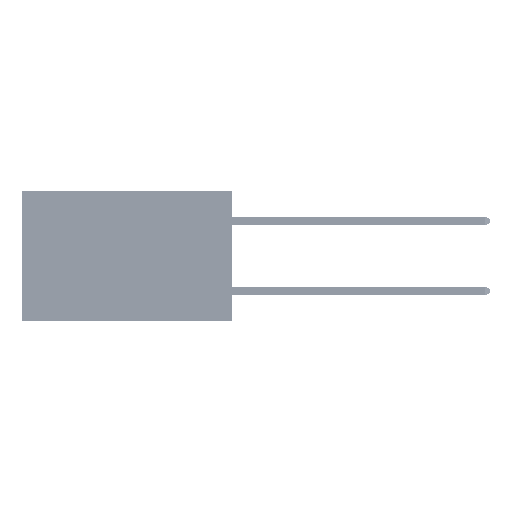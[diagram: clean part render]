
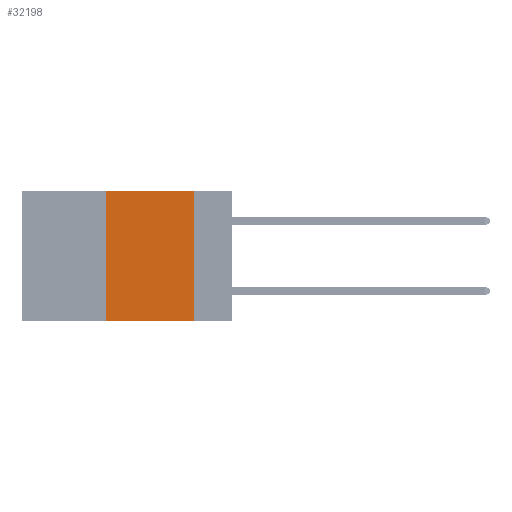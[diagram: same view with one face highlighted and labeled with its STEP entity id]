
A CAD part, left-side view. The second image highlights one B-rep face of the part: STEP entity #32198.
In plain terms, the highlighted planar face has unit normal (-1, 0, 0).
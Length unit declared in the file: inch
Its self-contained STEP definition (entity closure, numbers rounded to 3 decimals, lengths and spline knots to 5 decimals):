
#265 = CARTESIAN_POINT ( 'NONE',  ( 0., 0.11, -0.37 ) ) ;
#899 = EDGE_CURVE ( 'NONE', #46660, #8920, #6658, .T. ) ;
#1118 = VECTOR ( 'NONE', #45601, 39.37008 ) ;
#1864 = CARTESIAN_POINT ( 'NONE',  ( 0., 0.6, 0. ) ) ;
#2434 = DIRECTION ( 'NONE',  ( 0., 0., -1. ) ) ;
#5402 = VECTOR ( 'NONE', #34714, 39.37008 ) ;
#6658 = LINE ( 'NONE', #46500, #5402 ) ;
#8920 = VERTEX_POINT ( 'NONE', #45750 ) ;
#16286 = EDGE_LOOP ( 'NONE', ( #32082, #28455, #41812, #21680 ) ) ;
#16944 = VECTOR ( 'NONE', #51360, 39.37008 ) ;
#18183 = LINE ( 'NONE', #19348, #16944 ) ;
#19348 = CARTESIAN_POINT ( 'NONE',  ( 0., 0.6, 0. ) ) ;
#20403 = FACE_OUTER_BOUND ( 'NONE', #16286, .T. ) ;
#21680 = ORIENTED_EDGE ( 'NONE', *, *, #40168, .T. ) ;
#22173 = DIRECTION ( 'NONE',  ( 1., 0., 0. ) ) ;
#22852 = LINE ( 'NONE', #25361, #49208 ) ;
#23668 = LINE ( 'NONE', #29437, #1118 ) ;
#25361 = CARTESIAN_POINT ( 'NONE',  ( 0., 0.11, 0. ) ) ;
#26413 = CARTESIAN_POINT ( 'NONE',  ( 0., 0.11, 0. ) ) ;
#27241 = CARTESIAN_POINT ( 'NONE',  ( 0., 0.36, -0.37 ) ) ;
#28455 = ORIENTED_EDGE ( 'NONE', *, *, #44262, .F. ) ;
#29437 = CARTESIAN_POINT ( 'NONE',  ( 0., 0.6, -0.37 ) ) ;
#31424 = VERTEX_POINT ( 'NONE', #265 ) ;
#32082 = ORIENTED_EDGE ( 'NONE', *, *, #46419, .F. ) ;
#32198 = ADVANCED_FACE ( 'NONE', ( #20403 ), #41791, .F. ) ;
#32455 = AXIS2_PLACEMENT_3D ( 'NONE', #1864, #22173, #37898 ) ;
#34714 = DIRECTION ( 'NONE',  ( 0., 0., 1. ) ) ;
#37898 = DIRECTION ( 'NONE',  ( 0., 0., -1. ) ) ;
#40168 = EDGE_CURVE ( 'NONE', #46660, #31424, #23668, .T. ) ;
#40932 = VERTEX_POINT ( 'NONE', #26413 ) ;
#41791 = PLANE ( 'NONE',  #32455 ) ;
#41812 = ORIENTED_EDGE ( 'NONE', *, *, #899, .F. ) ;
#44262 = EDGE_CURVE ( 'NONE', #8920, #40932, #18183, .T. ) ;
#45601 = DIRECTION ( 'NONE',  ( 0., -1., 0. ) ) ;
#45750 = CARTESIAN_POINT ( 'NONE',  ( 0., 0.36, 0. ) ) ;
#46419 = EDGE_CURVE ( 'NONE', #40932, #31424, #22852, .T. ) ;
#46500 = CARTESIAN_POINT ( 'NONE',  ( 0., 0.36, 0. ) ) ;
#46660 = VERTEX_POINT ( 'NONE', #27241 ) ;
#49208 = VECTOR ( 'NONE', #2434, 39.37008 ) ;
#51360 = DIRECTION ( 'NONE',  ( 0., -1., 0. ) ) ;
